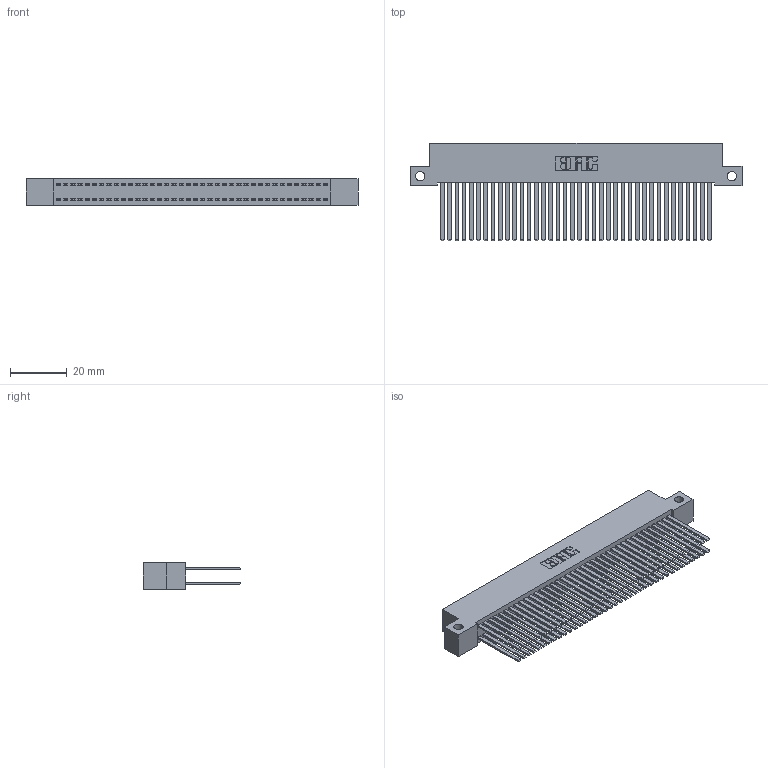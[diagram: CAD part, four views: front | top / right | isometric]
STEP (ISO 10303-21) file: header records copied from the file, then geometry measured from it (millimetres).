
FILE_DESCRIPTION (( 'STEP AP203' ), '1' );
FILE_NAME ('342-076-544-212.STEP', '2018-08-13T12:37:24', ( '' ), ( '' ), 'SwSTEP 2.0', 'SolidWorks 2016', '' );
FILE_SCHEMA (( 'CONFIG_CONTROL_DESIGN' ));
Length unit declared in the file: inch
Products named in the file (3): 345-292-001_345-293-144; 342-076-544-212; 342 Part_Side Mount
Assembly tree (77 placements, depth 2):
  342-076-544-212
    342 Part_Side Mount
    345-292-001_345-293-144  x76
Bounding box: 116.84 x 34.3 x 9.4 mm (x, y, z)
Volume: 11470.6 mm3; surface area: 21363.3 mm2
Topology: 77 solids, 77 shells, 3606 faces, 10711 edges, 7038 vertices
Faces by surface type: plane 2498, cylinder 1108
Entity records: 24651 total; most frequent: CARTESIAN_POINT 4086, ORIENTED_EDGE 4022, DIRECTION 3495, EDGE_CURVE 2011, LINE 1887, VECTOR 1887, VERTEX_POINT 1338, AXIS2_PLACEMENT_3D 804
